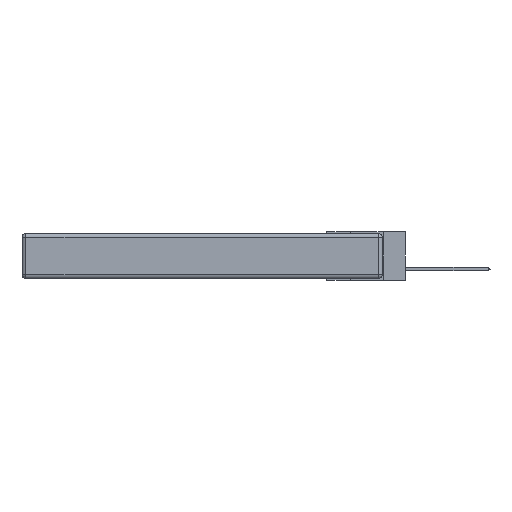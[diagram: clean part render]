
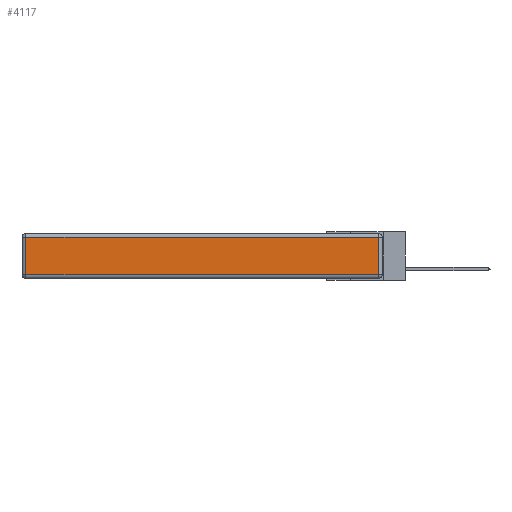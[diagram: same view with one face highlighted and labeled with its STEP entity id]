
A CAD part, left-side view. The second image highlights one B-rep face of the part: STEP entity #4117.
In plain terms, the highlighted planar face has unit normal (-1, 0, 0).
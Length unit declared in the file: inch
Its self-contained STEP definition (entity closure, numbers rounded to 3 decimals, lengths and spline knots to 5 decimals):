
#1739 = DIRECTION ( 'NONE',  ( 0., 1., 0. ) ) ;
#3205 = VECTOR ( 'NONE', #1739, 39.37008 ) ;
#3526 = VERTEX_POINT ( 'NONE', #24857 ) ;
#4117 = ADVANCED_FACE ( 'NONE', ( #28302 ), #6427, .T. ) ;
#4259 = DIRECTION ( 'NONE',  ( 0., 0., 1. ) ) ;
#6427 = PLANE ( 'NONE',  #26868 ) ;
#7828 = VECTOR ( 'NONE', #4259, 39.37008 ) ;
#13749 = LINE ( 'NONE', #21576, #19825 ) ;
#13799 = DIRECTION ( 'NONE',  ( -1., 0., 0. ) ) ;
#14552 = CARTESIAN_POINT ( 'NONE',  ( 0., 0.03, -0.343 ) ) ;
#15122 = CARTESIAN_POINT ( 'NONE',  ( 0., 0., -0.313 ) ) ;
#19275 = EDGE_LOOP ( 'NONE', ( #25098, #27588, #24523, #26993 ) ) ;
#19825 = VECTOR ( 'NONE', #21692, 39.37008 ) ;
#20799 = EDGE_CURVE ( 'NONE', #30219, #32153, #13749, .T. ) ;
#20932 = EDGE_CURVE ( 'NONE', #32153, #21512, #26703, .T. ) ;
#21413 = LINE ( 'NONE', #27992, #3205 ) ;
#21472 = CARTESIAN_POINT ( 'NONE',  ( 0., 0., -0.343 ) ) ;
#21512 = VERTEX_POINT ( 'NONE', #24550 ) ;
#21576 = CARTESIAN_POINT ( 'NONE',  ( 0., 2.72, -0.343 ) ) ;
#21692 = DIRECTION ( 'NONE',  ( 0., 0., -1. ) ) ;
#22372 = DIRECTION ( 'NONE',  ( 0., -1., 0. ) ) ;
#22810 = CARTESIAN_POINT ( 'NONE',  ( 0., 2.72, -0.03 ) ) ;
#24523 = ORIENTED_EDGE ( 'NONE', *, *, #33230, .T. ) ;
#24550 = CARTESIAN_POINT ( 'NONE',  ( 0., 0.03, -0.313 ) ) ;
#24857 = CARTESIAN_POINT ( 'NONE',  ( 0., 0.03, -0.03 ) ) ;
#25098 = ORIENTED_EDGE ( 'NONE', *, *, #20932, .T. ) ;
#26703 = LINE ( 'NONE', #15122, #30704 ) ;
#26739 = DIRECTION ( 'NONE',  ( 0., 0., 1. ) ) ;
#26868 = AXIS2_PLACEMENT_3D ( 'NONE', #21472, #13799, #26739 ) ;
#26993 = ORIENTED_EDGE ( 'NONE', *, *, #20799, .T. ) ;
#27588 = ORIENTED_EDGE ( 'NONE', *, *, #30061, .T. ) ;
#27992 = CARTESIAN_POINT ( 'NONE',  ( 0., 2.75, -0.03 ) ) ;
#28302 = FACE_OUTER_BOUND ( 'NONE', #19275, .T. ) ;
#28781 = CARTESIAN_POINT ( 'NONE',  ( 0., 2.72, -0.313 ) ) ;
#30061 = EDGE_CURVE ( 'NONE', #21512, #3526, #32129, .T. ) ;
#30219 = VERTEX_POINT ( 'NONE', #22810 ) ;
#30704 = VECTOR ( 'NONE', #22372, 39.37008 ) ;
#32129 = LINE ( 'NONE', #14552, #7828 ) ;
#32153 = VERTEX_POINT ( 'NONE', #28781 ) ;
#33230 = EDGE_CURVE ( 'NONE', #3526, #30219, #21413, .T. ) ;
